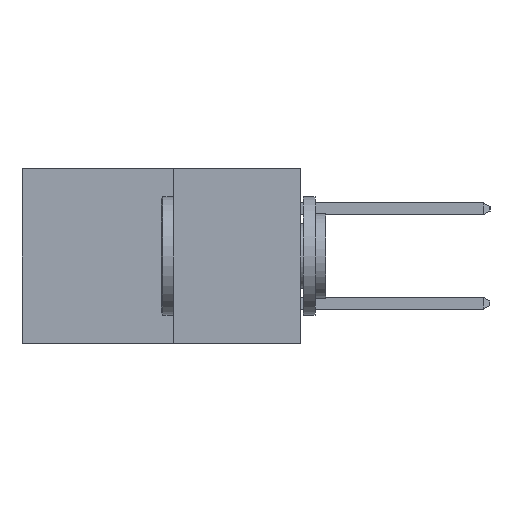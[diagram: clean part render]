
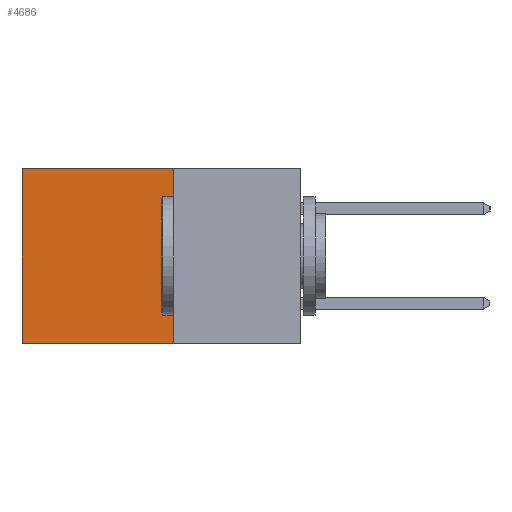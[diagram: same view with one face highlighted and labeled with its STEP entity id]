
A CAD part, left-side view. The second image highlights one B-rep face of the part: STEP entity #4686.
In plain terms, the highlighted planar face has unit normal (-1, 0, 0).
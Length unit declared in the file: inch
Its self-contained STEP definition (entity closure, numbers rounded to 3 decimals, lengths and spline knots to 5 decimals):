
#7 = DIRECTION ( 'NONE',  ( 0., 1., 0. ) ) ;
#47 = ORIENTED_EDGE ( 'NONE', *, *, #7638, .T. ) ;
#485 = DIRECTION ( 'NONE',  ( 0., 0., -1. ) ) ;
#727 = CARTESIAN_POINT ( 'NONE',  ( 0.277, 0.59, 0. ) ) ;
#1007 = VERTEX_POINT ( 'NONE', #3844 ) ;
#1213 = VECTOR ( 'NONE', #6489, 39.37008 ) ;
#1385 = LINE ( 'NONE', #4709, #8414 ) ;
#1690 = VECTOR ( 'NONE', #5839, 39.37008 ) ;
#1962 = EDGE_CURVE ( 'NONE', #2119, #6546, #5287, .T. ) ;
#2032 = ORIENTED_EDGE ( 'NONE', *, *, #4459, .T. ) ;
#2119 = VERTEX_POINT ( 'NONE', #8362 ) ;
#2441 = ORIENTED_EDGE ( 'NONE', *, *, #3757, .F. ) ;
#2586 = FACE_OUTER_BOUND ( 'NONE', #5309, .T. ) ;
#2797 = ORIENTED_EDGE ( 'NONE', *, *, #1962, .F. ) ;
#3757 = EDGE_CURVE ( 'NONE', #6546, #1007, #1385, .T. ) ;
#3844 = CARTESIAN_POINT ( 'NONE',  ( 0.277, 0.59, -0.37 ) ) ;
#4173 = CARTESIAN_POINT ( 'NONE',  ( 0.277, 0.59, -0.37 ) ) ;
#4459 = EDGE_CURVE ( 'NONE', #6098, #1007, #5128, .T. ) ;
#4686 = ADVANCED_FACE ( 'NONE', ( #2586 ), #7777, .F. ) ;
#4709 = CARTESIAN_POINT ( 'NONE',  ( 0.277, 0.27, -0.37 ) ) ;
#5007 = CARTESIAN_POINT ( 'NONE',  ( 0.277, 0.27, -0.37 ) ) ;
#5128 = LINE ( 'NONE', #4173, #1690 ) ;
#5163 = DIRECTION ( 'NONE',  ( 1., 0., 0. ) ) ;
#5287 = LINE ( 'NONE', #6230, #6214 ) ;
#5309 = EDGE_LOOP ( 'NONE', ( #2032, #2441, #2797, #47 ) ) ;
#5463 = CARTESIAN_POINT ( 'NONE',  ( 0.277, 0.27, -0.37 ) ) ;
#5812 = CARTESIAN_POINT ( 'NONE',  ( 0.277, 0.27, 0. ) ) ;
#5839 = DIRECTION ( 'NONE',  ( 0., 0., -1. ) ) ;
#6098 = VERTEX_POINT ( 'NONE', #727 ) ;
#6116 = AXIS2_PLACEMENT_3D ( 'NONE', #5007, #5163, #8646 ) ;
#6214 = VECTOR ( 'NONE', #485, 39.37008 ) ;
#6230 = CARTESIAN_POINT ( 'NONE',  ( 0.277, 0.27, -0.37 ) ) ;
#6489 = DIRECTION ( 'NONE',  ( 0., 1., 0. ) ) ;
#6546 = VERTEX_POINT ( 'NONE', #5463 ) ;
#7000 = LINE ( 'NONE', #5812, #1213 ) ;
#7638 = EDGE_CURVE ( 'NONE', #2119, #6098, #7000, .T. ) ;
#7777 = PLANE ( 'NONE',  #6116 ) ;
#8362 = CARTESIAN_POINT ( 'NONE',  ( 0.277, 0.27, 0. ) ) ;
#8414 = VECTOR ( 'NONE', #7, 39.37008 ) ;
#8646 = DIRECTION ( 'NONE',  ( 0., 0., -1. ) ) ;
